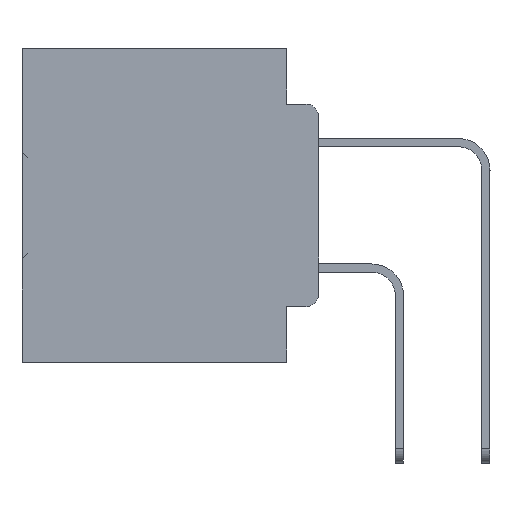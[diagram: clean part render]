
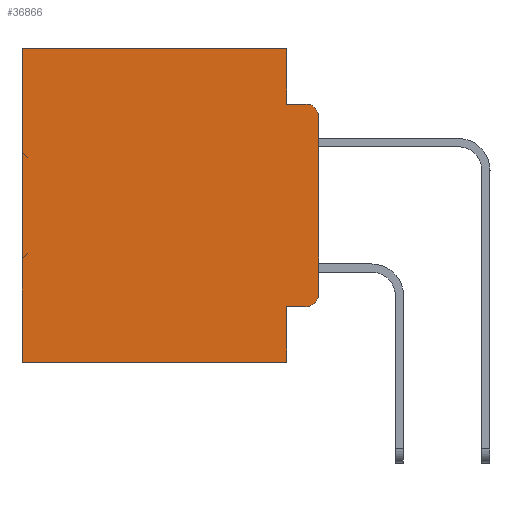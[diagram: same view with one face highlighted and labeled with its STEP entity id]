
A CAD part, left-side view. The second image highlights one B-rep face of the part: STEP entity #36866.
In plain terms, the highlighted planar face has unit normal (-1, 0, 0).
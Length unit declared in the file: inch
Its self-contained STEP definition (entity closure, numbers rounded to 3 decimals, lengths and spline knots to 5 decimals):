
#895 = VERTEX_POINT ( 'NONE', #22761 ) ;
#1424 = CARTESIAN_POINT ( 'NONE',  ( 0.298, 0.051, -0.0885 ) ) ;
#1948 = CARTESIAN_POINT ( 'NONE',  ( 0.298, 0.473, 0. ) ) ;
#2562 = ORIENTED_EDGE ( 'NONE', *, *, #6428, .F. ) ;
#2909 = DIRECTION ( 'NONE',  ( 0., 0., -1. ) ) ;
#3617 = ORIENTED_EDGE ( 'NONE', *, *, #5932, .F. ) ;
#3712 = CARTESIAN_POINT ( 'NONE',  ( 0.298, 0.02, -0.1085 ) ) ;
#5563 = EDGE_CURVE ( 'NONE', #11382, #27565, #13770, .T. ) ;
#5811 = LINE ( 'NONE', #7319, #21921 ) ;
#5932 = EDGE_CURVE ( 'NONE', #32360, #8929, #25657, .T. ) ;
#6428 = EDGE_CURVE ( 'NONE', #22213, #27565, #14209, .T. ) ;
#6773 = ORIENTED_EDGE ( 'NONE', *, *, #32224, .F. ) ;
#7319 = CARTESIAN_POINT ( 'NONE',  ( 0.298, 0., 0. ) ) ;
#7395 = CARTESIAN_POINT ( 'NONE',  ( 0.298, 0.02, -0.0885 ) ) ;
#7943 = CARTESIAN_POINT ( 'NONE',  ( 0.298, 0., -0.5 ) ) ;
#8516 = DIRECTION ( 'NONE',  ( 0., 0., -1. ) ) ;
#8903 = DIRECTION ( 'NONE',  ( -1., 0., 0. ) ) ;
#8929 = VERTEX_POINT ( 'NONE', #22258 ) ;
#9116 = PLANE ( 'NONE',  #12840 ) ;
#9129 = VECTOR ( 'NONE', #17181, 39.37008 ) ;
#10055 = DIRECTION ( 'NONE',  ( 0., 0., -1. ) ) ;
#10302 = CARTESIAN_POINT ( 'NONE',  ( 0.298, 0.051, -0.5 ) ) ;
#10438 = EDGE_CURVE ( 'NONE', #11382, #28233, #14633, .T. ) ;
#10705 = CARTESIAN_POINT ( 'NONE',  ( 0.298, 0.051, 0. ) ) ;
#11382 = VERTEX_POINT ( 'NONE', #16109 ) ;
#11389 = VECTOR ( 'NONE', #23459, 39.37008 ) ;
#11433 = EDGE_CURVE ( 'NONE', #895, #24446, #17439, .T. ) ;
#12840 = AXIS2_PLACEMENT_3D ( 'NONE', #21047, #30504, #2909 ) ;
#13728 = ORIENTED_EDGE ( 'NONE', *, *, #10438, .F. ) ;
#13770 = CIRCLE ( 'NONE', #19423, 0.02 ) ;
#14209 = LINE ( 'NONE', #25974, #37518 ) ;
#14633 = LINE ( 'NONE', #20719, #20809 ) ;
#15353 = FACE_OUTER_BOUND ( 'NONE', #20564, .T. ) ;
#16109 = CARTESIAN_POINT ( 'NONE',  ( 0.298, 0., -0.1085 ) ) ;
#17181 = DIRECTION ( 'NONE',  ( 0., 0., -1. ) ) ;
#17275 = LINE ( 'NONE', #28161, #21078 ) ;
#17330 = ORIENTED_EDGE ( 'NONE', *, *, #36489, .T. ) ;
#17439 = LINE ( 'NONE', #31167, #26970 ) ;
#17525 = EDGE_CURVE ( 'NONE', #895, #32360, #29586, .T. ) ;
#17654 = ORIENTED_EDGE ( 'NONE', *, *, #17525, .F. ) ;
#18148 = ORIENTED_EDGE ( 'NONE', *, *, #5563, .T. ) ;
#19172 = VECTOR ( 'NONE', #31828, 39.37008 ) ;
#19423 = AXIS2_PLACEMENT_3D ( 'NONE', #3712, #25201, #10055 ) ;
#19446 = EDGE_CURVE ( 'NONE', #29255, #22360, #5811, .T. ) ;
#20564 = EDGE_LOOP ( 'NONE', ( #13728, #18148, #2562, #6773, #25918, #17330, #3617, #17654, #33800, #39079 ) ) ;
#20719 = CARTESIAN_POINT ( 'NONE',  ( 0.298, 0., 0. ) ) ;
#20809 = VECTOR ( 'NONE', #26379, 39.37008 ) ;
#21047 = CARTESIAN_POINT ( 'NONE',  ( 0.298, 0., 0. ) ) ;
#21078 = VECTOR ( 'NONE', #28690, 39.37008 ) ;
#21921 = VECTOR ( 'NONE', #37338, 39.37008 ) ;
#22213 = VERTEX_POINT ( 'NONE', #1424 ) ;
#22258 = CARTESIAN_POINT ( 'NONE',  ( 0.298, 0.473, -0.5 ) ) ;
#22360 = VERTEX_POINT ( 'NONE', #1948 ) ;
#22403 = CARTESIAN_POINT ( 'NONE',  ( 0.298, 0.051, 0. ) ) ;
#22514 = EDGE_CURVE ( 'NONE', #24446, #28233, #35088, .T. ) ;
#22761 = CARTESIAN_POINT ( 'NONE',  ( 0.298, 0.051, -0.4115 ) ) ;
#23431 = CARTESIAN_POINT ( 'NONE',  ( 0.298, 0.051, 0. ) ) ;
#23459 = DIRECTION ( 'NONE',  ( 0., 1., 0. ) ) ;
#23937 = LINE ( 'NONE', #10705, #19172 ) ;
#24446 = VERTEX_POINT ( 'NONE', #29382 ) ;
#25201 = DIRECTION ( 'NONE',  ( -1., 0., 0. ) ) ;
#25324 = DIRECTION ( 'NONE',  ( 0., -1., 0. ) ) ;
#25657 = LINE ( 'NONE', #7943, #11389 ) ;
#25918 = ORIENTED_EDGE ( 'NONE', *, *, #19446, .T. ) ;
#25974 = CARTESIAN_POINT ( 'NONE',  ( 0.298, 0.051, -0.0885 ) ) ;
#26379 = DIRECTION ( 'NONE',  ( 0., 0., -1. ) ) ;
#26741 = CARTESIAN_POINT ( 'NONE',  ( 0.298, 0.02, -0.3915 ) ) ;
#26970 = VECTOR ( 'NONE', #25324, 39.37008 ) ;
#27565 = VERTEX_POINT ( 'NONE', #7395 ) ;
#28161 = CARTESIAN_POINT ( 'NONE',  ( 0.298, 0.473, 0. ) ) ;
#28233 = VERTEX_POINT ( 'NONE', #29582 ) ;
#28690 = DIRECTION ( 'NONE',  ( 0., 0., -1. ) ) ;
#29255 = VERTEX_POINT ( 'NONE', #22403 ) ;
#29302 = DIRECTION ( 'NONE',  ( 0., -1., 0. ) ) ;
#29382 = CARTESIAN_POINT ( 'NONE',  ( 0.298, 0.02, -0.4115 ) ) ;
#29582 = CARTESIAN_POINT ( 'NONE',  ( 0.298, 0., -0.3915 ) ) ;
#29586 = LINE ( 'NONE', #23431, #9129 ) ;
#30504 = DIRECTION ( 'NONE',  ( 1., 0., 0. ) ) ;
#31167 = CARTESIAN_POINT ( 'NONE',  ( 0.298, 0.051, -0.4115 ) ) ;
#31828 = DIRECTION ( 'NONE',  ( 0., 0., -1. ) ) ;
#32224 = EDGE_CURVE ( 'NONE', #29255, #22213, #23937, .T. ) ;
#32360 = VERTEX_POINT ( 'NONE', #10302 ) ;
#33800 = ORIENTED_EDGE ( 'NONE', *, *, #11433, .T. ) ;
#34212 = AXIS2_PLACEMENT_3D ( 'NONE', #26741, #8903, #8516 ) ;
#35088 = CIRCLE ( 'NONE', #34212, 0.02 ) ;
#36489 = EDGE_CURVE ( 'NONE', #22360, #8929, #17275, .T. ) ;
#36866 = ADVANCED_FACE ( 'NONE', ( #15353 ), #9116, .F. ) ;
#37338 = DIRECTION ( 'NONE',  ( 0., 1., 0. ) ) ;
#37518 = VECTOR ( 'NONE', #29302, 39.37008 ) ;
#39079 = ORIENTED_EDGE ( 'NONE', *, *, #22514, .T. ) ;
